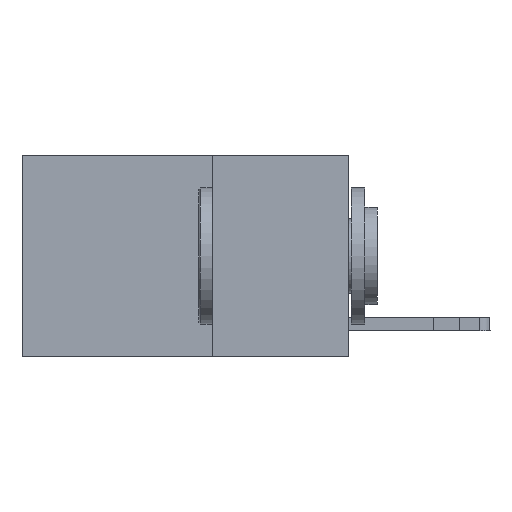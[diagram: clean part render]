
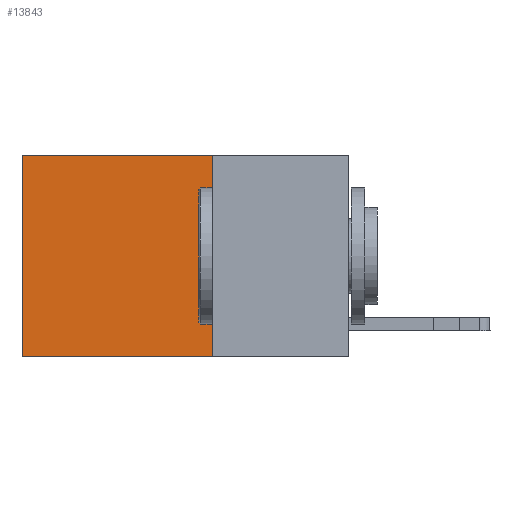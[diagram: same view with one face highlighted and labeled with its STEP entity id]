
A CAD part, left-side view. The second image highlights one B-rep face of the part: STEP entity #13843.
In plain terms, the highlighted planar face has unit normal (-1, 0, 0).
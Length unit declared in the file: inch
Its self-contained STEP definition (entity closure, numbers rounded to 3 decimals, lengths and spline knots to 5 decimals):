
#390 = VERTEX_POINT ( 'NONE', #22427 ) ;
#494 = CARTESIAN_POINT ( 'NONE',  ( 0.2625, 0.25, 0. ) ) ;
#1646 = LINE ( 'NONE', #10438, #14530 ) ;
#1748 = EDGE_CURVE ( 'NONE', #14447, #390, #11907, .T. ) ;
#2235 = CARTESIAN_POINT ( 'NONE',  ( 0.2625, 0.25, 0. ) ) ;
#3399 = VECTOR ( 'NONE', #7559, 39.37008 ) ;
#4415 = VECTOR ( 'NONE', #17303, 39.37008 ) ;
#4719 = CARTESIAN_POINT ( 'NONE',  ( 0.2625, 0.25, 0. ) ) ;
#4903 = DIRECTION ( 'NONE',  ( 0., 0., -1. ) ) ;
#5887 = DIRECTION ( 'NONE',  ( 0., 0., -1. ) ) ;
#7499 = DIRECTION ( 'NONE',  ( 0., 0., -1. ) ) ;
#7559 = DIRECTION ( 'NONE',  ( 0., 1., 0. ) ) ;
#7611 = ORIENTED_EDGE ( 'NONE', *, *, #22372, .T. ) ;
#8873 = VERTEX_POINT ( 'NONE', #18769 ) ;
#9686 = EDGE_CURVE ( 'NONE', #14447, #21968, #21158, .T. ) ;
#10002 = EDGE_LOOP ( 'NONE', ( #7611, #12977, #20394, #18408 ) ) ;
#10401 = EDGE_CURVE ( 'NONE', #21968, #8873, #14065, .T. ) ;
#10438 = CARTESIAN_POINT ( 'NONE',  ( 0.2625, 0.6, 0. ) ) ;
#11907 = LINE ( 'NONE', #22187, #4415 ) ;
#12346 = CARTESIAN_POINT ( 'NONE',  ( 0.2625, 0.25, -0.37 ) ) ;
#12664 = VECTOR ( 'NONE', #7499, 39.37008 ) ;
#12977 = ORIENTED_EDGE ( 'NONE', *, *, #10401, .F. ) ;
#13757 = AXIS2_PLACEMENT_3D ( 'NONE', #4719, #15207, #5887 ) ;
#13843 = ADVANCED_FACE ( 'NONE', ( #17671 ), #18561, .F. ) ;
#13883 = CARTESIAN_POINT ( 'NONE',  ( 0.2625, 0.25, -0.37 ) ) ;
#14065 = LINE ( 'NONE', #12346, #3399 ) ;
#14447 = VERTEX_POINT ( 'NONE', #494 ) ;
#14530 = VECTOR ( 'NONE', #4903, 39.37008 ) ;
#15207 = DIRECTION ( 'NONE',  ( 1., 0., 0. ) ) ;
#17303 = DIRECTION ( 'NONE',  ( 0., 1., 0. ) ) ;
#17671 = FACE_OUTER_BOUND ( 'NONE', #10002, .T. ) ;
#18408 = ORIENTED_EDGE ( 'NONE', *, *, #1748, .T. ) ;
#18561 = PLANE ( 'NONE',  #13757 ) ;
#18769 = CARTESIAN_POINT ( 'NONE',  ( 0.2625, 0.6, -0.37 ) ) ;
#20394 = ORIENTED_EDGE ( 'NONE', *, *, #9686, .F. ) ;
#21158 = LINE ( 'NONE', #2235, #12664 ) ;
#21968 = VERTEX_POINT ( 'NONE', #13883 ) ;
#22187 = CARTESIAN_POINT ( 'NONE',  ( 0.2625, 0.25, 0. ) ) ;
#22372 = EDGE_CURVE ( 'NONE', #390, #8873, #1646, .T. ) ;
#22427 = CARTESIAN_POINT ( 'NONE',  ( 0.2625, 0.6, 0. ) ) ;
